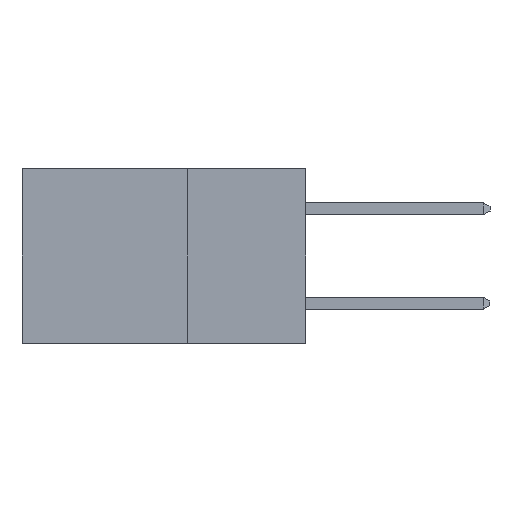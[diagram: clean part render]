
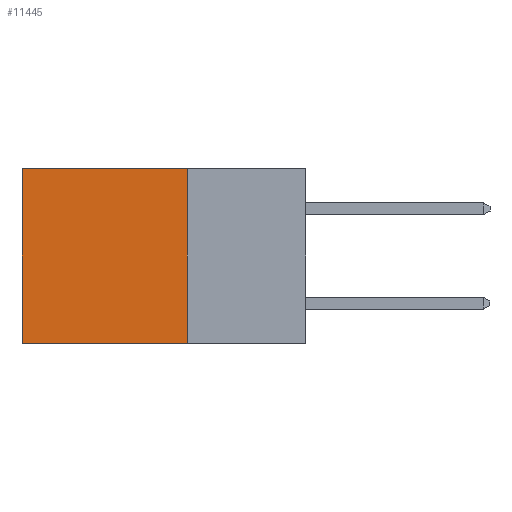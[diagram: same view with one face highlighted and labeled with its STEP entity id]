
A CAD part, left-side view. The second image highlights one B-rep face of the part: STEP entity #11445.
In plain terms, the highlighted planar face has unit normal (-1, 0, 0).
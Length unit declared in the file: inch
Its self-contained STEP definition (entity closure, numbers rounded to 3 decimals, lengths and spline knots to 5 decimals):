
#287 = CARTESIAN_POINT ( 'NONE',  ( 0.298, 0.6, 0. ) ) ;
#977 = VECTOR ( 'NONE', #10302, 39.37008 ) ;
#1008 = EDGE_CURVE ( 'NONE', #3588, #1291, #5632, .T. ) ;
#1092 = ORIENTED_EDGE ( 'NONE', *, *, #7161, .T. ) ;
#1291 = VERTEX_POINT ( 'NONE', #10767 ) ;
#1621 = ORIENTED_EDGE ( 'NONE', *, *, #3052, .T. ) ;
#1762 = VERTEX_POINT ( 'NONE', #3161 ) ;
#1959 = DIRECTION ( 'NONE',  ( 0., 0., -1. ) ) ;
#2248 = CARTESIAN_POINT ( 'NONE',  ( 0.298, 0.25, -0.37 ) ) ;
#2583 = ORIENTED_EDGE ( 'NONE', *, *, #11732, .F. ) ;
#2869 = PLANE ( 'NONE',  #3233 ) ;
#2979 = CARTESIAN_POINT ( 'NONE',  ( 0.298, 0.25, 0. ) ) ;
#3052 = EDGE_CURVE ( 'NONE', #1762, #11501, #6011, .T. ) ;
#3161 = CARTESIAN_POINT ( 'NONE',  ( 0.298, 0.6, 0. ) ) ;
#3233 = AXIS2_PLACEMENT_3D ( 'NONE', #11814, #9201, #3882 ) ;
#3267 = DIRECTION ( 'NONE',  ( 0., 1., 0. ) ) ;
#3534 = EDGE_LOOP ( 'NONE', ( #1621, #2583, #3685, #1092 ) ) ;
#3588 = VERTEX_POINT ( 'NONE', #9439 ) ;
#3685 = ORIENTED_EDGE ( 'NONE', *, *, #1008, .F. ) ;
#3882 = DIRECTION ( 'NONE',  ( 0., 0., -1. ) ) ;
#5255 = CARTESIAN_POINT ( 'NONE',  ( 0.298, 0.25, 0. ) ) ;
#5597 = LINE ( 'NONE', #2248, #7675 ) ;
#5632 = LINE ( 'NONE', #5255, #9498 ) ;
#6011 = LINE ( 'NONE', #287, #977 ) ;
#7161 = EDGE_CURVE ( 'NONE', #3588, #1762, #9813, .T. ) ;
#7675 = VECTOR ( 'NONE', #3267, 39.37008 ) ;
#7765 = VECTOR ( 'NONE', #8425, 39.37008 ) ;
#8107 = FACE_OUTER_BOUND ( 'NONE', #3534, .T. ) ;
#8409 = CARTESIAN_POINT ( 'NONE',  ( 0.298, 0.6, -0.37 ) ) ;
#8425 = DIRECTION ( 'NONE',  ( 0., 1., 0. ) ) ;
#9201 = DIRECTION ( 'NONE',  ( 1., 0., 0. ) ) ;
#9439 = CARTESIAN_POINT ( 'NONE',  ( 0.298, 0.25, 0. ) ) ;
#9498 = VECTOR ( 'NONE', #1959, 39.37008 ) ;
#9813 = LINE ( 'NONE', #2979, #7765 ) ;
#10302 = DIRECTION ( 'NONE',  ( 0., 0., -1. ) ) ;
#10767 = CARTESIAN_POINT ( 'NONE',  ( 0.298, 0.25, -0.37 ) ) ;
#11445 = ADVANCED_FACE ( 'NONE', ( #8107 ), #2869, .F. ) ;
#11501 = VERTEX_POINT ( 'NONE', #8409 ) ;
#11732 = EDGE_CURVE ( 'NONE', #1291, #11501, #5597, .T. ) ;
#11814 = CARTESIAN_POINT ( 'NONE',  ( 0.298, 0.25, 0. ) ) ;
